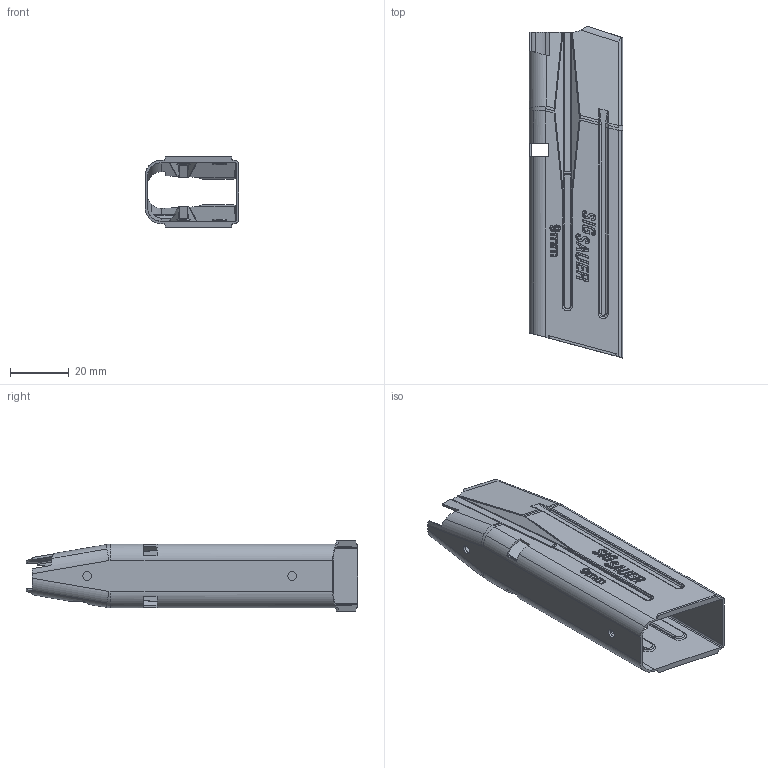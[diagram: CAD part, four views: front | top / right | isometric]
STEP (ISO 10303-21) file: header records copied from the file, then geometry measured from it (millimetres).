
FILE_DESCRIPTION (( 'STEP AP214' ), '1' );
FILE_NAME ('Magazine Tube - Copy.step', '2014-07-30T19:46:21', ( 'WarFairy' ), ( '' ), 'SwSTEP 2.0', 'SolidWorks 2013', '' );
FILE_SCHEMA (( 'AUTOMOTIVE_DESIGN' ));
Length unit declared in the file: millimetre
Products named in the file (1): Magazine Tube - Copy
Bounding box: 32.11 x 113.49 x 24 mm (x, y, z)
Volume: 8418 mm3; surface area: 21278.4 mm2
Topology: 1 solids, 1 shells, 1026 faces, 2790 edges, 1798 vertices
Faces by surface type: plane 453, bspline 299, cylinder 246, torus 16, sphere 12
Entity records: 36028 total; most frequent: CARTESIAN_POINT 12880, ORIENTED_EDGE 5558, DIRECTION 3506, EDGE_CURVE 2779, VERTEX_POINT 1798, LINE 1656, VECTOR 1656, EDGE_LOOP 1085
